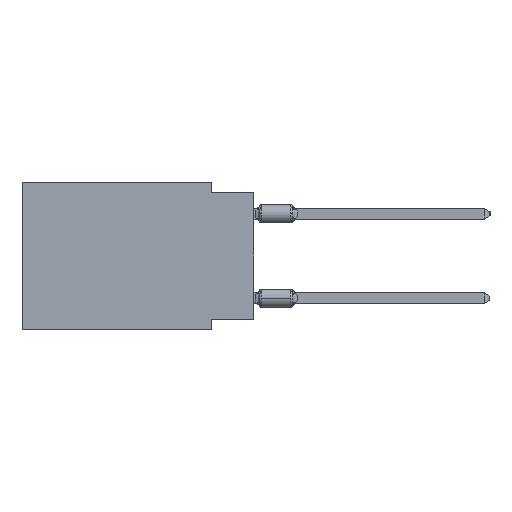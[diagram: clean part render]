
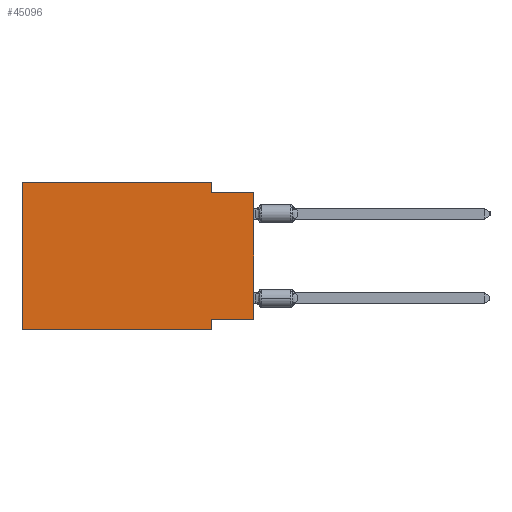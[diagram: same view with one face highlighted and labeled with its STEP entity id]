
A CAD part, left-side view. The second image highlights one B-rep face of the part: STEP entity #45096.
In plain terms, the highlighted planar face has unit normal (-1, 0, 0).
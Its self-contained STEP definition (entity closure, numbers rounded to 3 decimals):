
#1117 = DIRECTION ( 'NONE',  ( 0., -1., 0. ) ) ;
#1171 = DIRECTION ( 'NONE',  ( 0., -1., 0. ) ) ;
#1368 = VERTEX_POINT ( 'NONE', #32011 ) ;
#1470 = LINE ( 'NONE', #48986, #9483 ) ;
#1775 = CARTESIAN_POINT ( 'NONE',  ( 0., 13.97, -8.89 ) ) ;
#2205 = VERTEX_POINT ( 'NONE', #26613 ) ;
#4609 = CARTESIAN_POINT ( 'NONE',  ( 0., 2.54, -8.89 ) ) ;
#4845 = PLANE ( 'NONE',  #35787 ) ;
#5515 = VECTOR ( 'NONE', #50058, 1000. ) ;
#6113 = CARTESIAN_POINT ( 'NONE',  ( 0., 13.97, 0. ) ) ;
#6833 = EDGE_CURVE ( 'NONE', #60544, #1368, #55314, .T. ) ;
#8389 = VERTEX_POINT ( 'NONE', #25602 ) ;
#8887 = ORIENTED_EDGE ( 'NONE', *, *, #25360, .F. ) ;
#9483 = VECTOR ( 'NONE', #15763, 1000. ) ;
#9702 = EDGE_CURVE ( 'NONE', #2205, #8389, #55376, .T. ) ;
#9893 = EDGE_CURVE ( 'NONE', #28401, #35873, #42959, .T. ) ;
#11640 = CARTESIAN_POINT ( 'NONE',  ( 0., 0., -0.635 ) ) ;
#11965 = VERTEX_POINT ( 'NONE', #58538 ) ;
#12780 = EDGE_CURVE ( 'NONE', #28401, #18316, #1470, .T. ) ;
#14486 = FACE_OUTER_BOUND ( 'NONE', #23962, .T. ) ;
#14551 = LINE ( 'NONE', #4609, #16233 ) ;
#15763 = DIRECTION ( 'NONE',  ( 0., 0., 1. ) ) ;
#16233 = VECTOR ( 'NONE', #61121, 1000. ) ;
#18316 = VERTEX_POINT ( 'NONE', #11640 ) ;
#18349 = VECTOR ( 'NONE', #45883, 1000. ) ;
#20648 = ORIENTED_EDGE ( 'NONE', *, *, #12780, .T. ) ;
#20861 = ORIENTED_EDGE ( 'NONE', *, *, #46405, .F. ) ;
#20982 = CARTESIAN_POINT ( 'NONE',  ( 0., 0., -0.635 ) ) ;
#21270 = CARTESIAN_POINT ( 'NONE',  ( 0., 0., -8.255 ) ) ;
#23962 = EDGE_LOOP ( 'NONE', ( #20648, #20861, #43298, #57736, #8887, #27243, #34528, #32607 ) ) ;
#25021 = LINE ( 'NONE', #20982, #43027 ) ;
#25360 = EDGE_CURVE ( 'NONE', #2205, #11965, #48352, .T. ) ;
#25602 = CARTESIAN_POINT ( 'NONE',  ( 0., 2.54, -8.89 ) ) ;
#26613 = CARTESIAN_POINT ( 'NONE',  ( 0., 13.97, -8.89 ) ) ;
#27243 = ORIENTED_EDGE ( 'NONE', *, *, #9702, .T. ) ;
#27374 = CARTESIAN_POINT ( 'NONE',  ( 0., 2.54, 0. ) ) ;
#28401 = VERTEX_POINT ( 'NONE', #21270 ) ;
#29588 = DIRECTION ( 'NONE',  ( 0., 1., 0. ) ) ;
#29707 = CARTESIAN_POINT ( 'NONE',  ( 0., 2.54, -8.255 ) ) ;
#32011 = CARTESIAN_POINT ( 'NONE',  ( 0., 2.54, -0.635 ) ) ;
#32607 = ORIENTED_EDGE ( 'NONE', *, *, #9893, .F. ) ;
#33264 = EDGE_CURVE ( 'NONE', #11965, #60544, #56421, .T. ) ;
#34528 = ORIENTED_EDGE ( 'NONE', *, *, #43433, .F. ) ;
#35787 = AXIS2_PLACEMENT_3D ( 'NONE', #42747, #52362, #56075 ) ;
#35873 = VERTEX_POINT ( 'NONE', #29707 ) ;
#42747 = CARTESIAN_POINT ( 'NONE',  ( 0., 13.97, 0. ) ) ;
#42959 = LINE ( 'NONE', #44190, #54250 ) ;
#43027 = VECTOR ( 'NONE', #1117, 1000. ) ;
#43298 = ORIENTED_EDGE ( 'NONE', *, *, #6833, .F. ) ;
#43433 = EDGE_CURVE ( 'NONE', #35873, #8389, #14551, .T. ) ;
#44190 = CARTESIAN_POINT ( 'NONE',  ( 0., 0., -8.255 ) ) ;
#45096 = ADVANCED_FACE ( 'NONE', ( #14486 ), #4845, .F. ) ;
#45883 = DIRECTION ( 'NONE',  ( 0., -1., 0. ) ) ;
#46242 = CARTESIAN_POINT ( 'NONE',  ( 0., 2.54, 0. ) ) ;
#46405 = EDGE_CURVE ( 'NONE', #1368, #18316, #25021, .T. ) ;
#46497 = CARTESIAN_POINT ( 'NONE',  ( 0., 13.97, 0. ) ) ;
#46598 = VECTOR ( 'NONE', #58884, 1000. ) ;
#48352 = LINE ( 'NONE', #6113, #46598 ) ;
#48986 = CARTESIAN_POINT ( 'NONE',  ( 0., 0., 0. ) ) ;
#50058 = DIRECTION ( 'NONE',  ( 0., 0., -1. ) ) ;
#52362 = DIRECTION ( 'NONE',  ( 1., 0., 0. ) ) ;
#54250 = VECTOR ( 'NONE', #29588, 1000. ) ;
#55314 = LINE ( 'NONE', #27374, #5515 ) ;
#55376 = LINE ( 'NONE', #1775, #61198 ) ;
#56075 = DIRECTION ( 'NONE',  ( 0., 0., -1. ) ) ;
#56421 = LINE ( 'NONE', #46497, #18349 ) ;
#57736 = ORIENTED_EDGE ( 'NONE', *, *, #33264, .F. ) ;
#58538 = CARTESIAN_POINT ( 'NONE',  ( 0., 13.97, 0. ) ) ;
#58884 = DIRECTION ( 'NONE',  ( 0., 0., 1. ) ) ;
#60544 = VERTEX_POINT ( 'NONE', #46242 ) ;
#61121 = DIRECTION ( 'NONE',  ( 0., 0., -1. ) ) ;
#61198 = VECTOR ( 'NONE', #1171, 1000. ) ;
